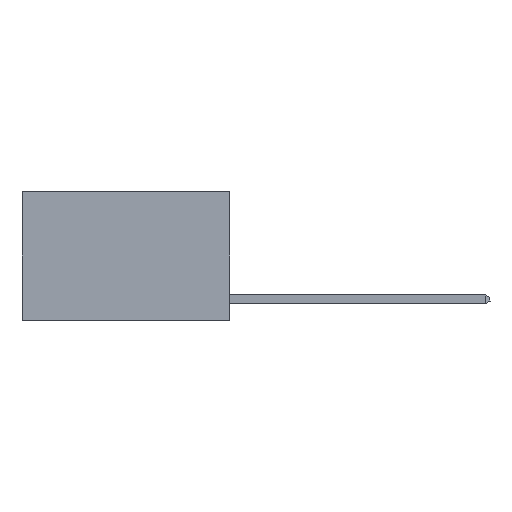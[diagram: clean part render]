
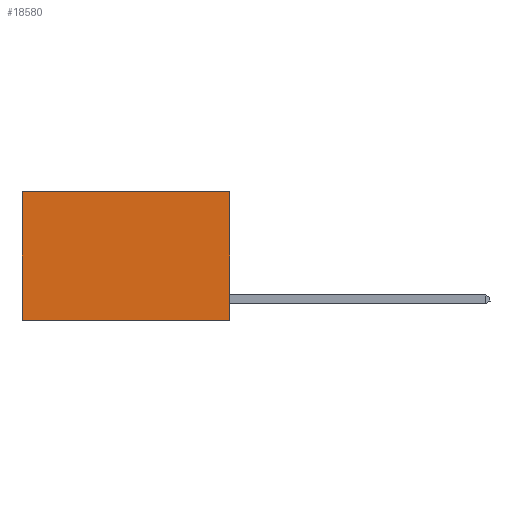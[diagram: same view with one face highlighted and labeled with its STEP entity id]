
A CAD part, left-side view. The second image highlights one B-rep face of the part: STEP entity #18580.
In plain terms, the highlighted planar face has unit normal (-1, 0, 0).
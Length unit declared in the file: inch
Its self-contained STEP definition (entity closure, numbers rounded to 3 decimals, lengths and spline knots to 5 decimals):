
#1473 = CARTESIAN_POINT ( 'NONE',  ( 0.2625, 0., 0. ) ) ;
#1537 = LINE ( 'NONE', #13434, #13536 ) ;
#2261 = CARTESIAN_POINT ( 'NONE',  ( 0.2625, 0., 0. ) ) ;
#2749 = EDGE_LOOP ( 'NONE', ( #5793, #25745, #13155, #13665 ) ) ;
#2891 = FACE_OUTER_BOUND ( 'NONE', #2749, .T. ) ;
#2901 = VECTOR ( 'NONE', #10498, 39.37008 ) ;
#4447 = CARTESIAN_POINT ( 'NONE',  ( 0.2625, 0., 0. ) ) ;
#5701 = DIRECTION ( 'NONE',  ( 0., 0., -1. ) ) ;
#5793 = ORIENTED_EDGE ( 'NONE', *, *, #14687, .T. ) ;
#6541 = DIRECTION ( 'NONE',  ( 1., 0., 0. ) ) ;
#6844 = VERTEX_POINT ( 'NONE', #12778 ) ;
#7675 = EDGE_CURVE ( 'NONE', #12626, #6844, #20154, .T. ) ;
#8853 = VECTOR ( 'NONE', #9442, 39.37008 ) ;
#9039 = CARTESIAN_POINT ( 'NONE',  ( 0.2625, 0., 0. ) ) ;
#9442 = DIRECTION ( 'NONE',  ( 0., 1., 0. ) ) ;
#9666 = VECTOR ( 'NONE', #12884, 39.37008 ) ;
#10498 = DIRECTION ( 'NONE',  ( 0., 0., -1. ) ) ;
#11127 = AXIS2_PLACEMENT_3D ( 'NONE', #4447, #6541, #14917 ) ;
#11652 = LINE ( 'NONE', #1473, #8853 ) ;
#11716 = EDGE_CURVE ( 'NONE', #6844, #24901, #20976, .T. ) ;
#12325 = EDGE_CURVE ( 'NONE', #12626, #16793, #11652, .T. ) ;
#12626 = VERTEX_POINT ( 'NONE', #9039 ) ;
#12778 = CARTESIAN_POINT ( 'NONE',  ( 0.2625, 0., -0.37 ) ) ;
#12884 = DIRECTION ( 'NONE',  ( 0., 1., 0. ) ) ;
#12951 = PLANE ( 'NONE',  #11127 ) ;
#13155 = ORIENTED_EDGE ( 'NONE', *, *, #7675, .F. ) ;
#13434 = CARTESIAN_POINT ( 'NONE',  ( 0.2625, 0.6, 0. ) ) ;
#13536 = VECTOR ( 'NONE', #5701, 39.37008 ) ;
#13665 = ORIENTED_EDGE ( 'NONE', *, *, #12325, .T. ) ;
#14687 = EDGE_CURVE ( 'NONE', #16793, #24901, #1537, .T. ) ;
#14917 = DIRECTION ( 'NONE',  ( 0., 0., -1. ) ) ;
#16793 = VERTEX_POINT ( 'NONE', #22920 ) ;
#18580 = ADVANCED_FACE ( 'NONE', ( #2891 ), #12951, .F. ) ;
#18767 = CARTESIAN_POINT ( 'NONE',  ( 0.2625, 0., -0.37 ) ) ;
#20154 = LINE ( 'NONE', #2261, #2901 ) ;
#20976 = LINE ( 'NONE', #18767, #9666 ) ;
#22920 = CARTESIAN_POINT ( 'NONE',  ( 0.2625, 0.6, 0. ) ) ;
#24901 = VERTEX_POINT ( 'NONE', #25011 ) ;
#25011 = CARTESIAN_POINT ( 'NONE',  ( 0.2625, 0.6, -0.37 ) ) ;
#25745 = ORIENTED_EDGE ( 'NONE', *, *, #11716, .F. ) ;
